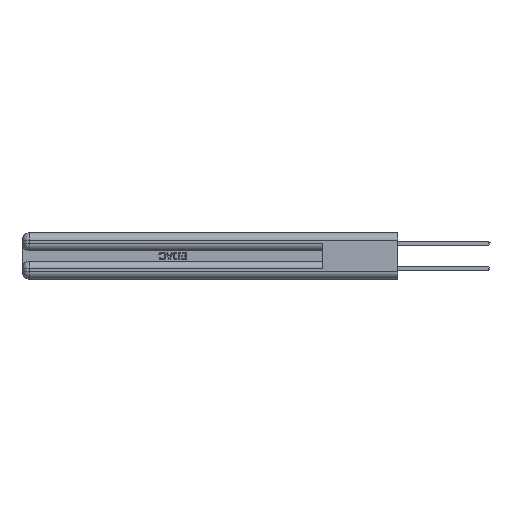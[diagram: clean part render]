
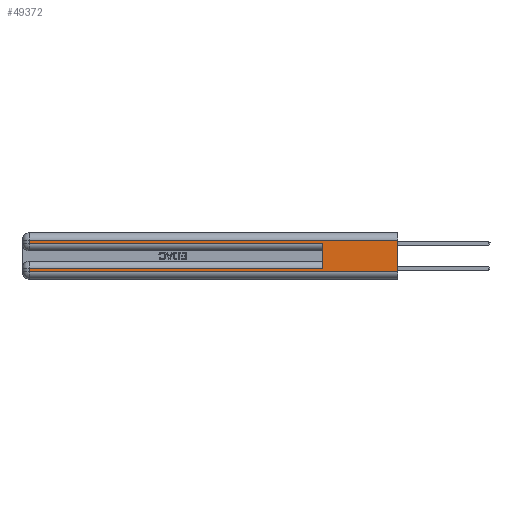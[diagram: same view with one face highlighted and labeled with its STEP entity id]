
A CAD part, left-side view. The second image highlights one B-rep face of the part: STEP entity #49372.
In plain terms, the highlighted planar face has unit normal (-1, 0, 0).
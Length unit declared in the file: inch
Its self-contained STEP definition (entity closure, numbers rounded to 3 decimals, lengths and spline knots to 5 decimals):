
#374 = EDGE_CURVE ( 'NONE', #12923, #14747, #52393, .T. ) ;
#534 = EDGE_CURVE ( 'NONE', #12923, #925, #26849, .T. ) ;
#585 = CARTESIAN_POINT ( 'NONE',  ( 0., 0., 0.37 ) ) ;
#694 = VECTOR ( 'NONE', #835, 39.37008 ) ;
#835 = DIRECTION ( 'NONE',  ( 0., 0., -1. ) ) ;
#925 = VERTEX_POINT ( 'NONE', #38892 ) ;
#1058 = LINE ( 'NONE', #45778, #47148 ) ;
#1672 = DIRECTION ( 'NONE',  ( 0., -1., 0. ) ) ;
#3564 = DIRECTION ( 'NONE',  ( 0., 1., 0. ) ) ;
#4572 = CARTESIAN_POINT ( 'NONE',  ( 0., 2.94, 0.37 ) ) ;
#5082 = CARTESIAN_POINT ( 'NONE',  ( 0., 0., 0.31 ) ) ;
#5516 = EDGE_CURVE ( 'NONE', #925, #50836, #44206, .T. ) ;
#7382 = DIRECTION ( 'NONE',  ( 0., 1., 0. ) ) ;
#8283 = VECTOR ( 'NONE', #7382, 39.37008 ) ;
#8948 = VECTOR ( 'NONE', #32881, 39.37008 ) ;
#10484 = ORIENTED_EDGE ( 'NONE', *, *, #16771, .F. ) ;
#10670 = EDGE_CURVE ( 'NONE', #12885, #26921, #10829, .T. ) ;
#10829 = LINE ( 'NONE', #48444, #51081 ) ;
#10860 = VECTOR ( 'NONE', #1672, 39.37008 ) ;
#12379 = EDGE_CURVE ( 'NONE', #45202, #14747, #41952, .T. ) ;
#12885 = VERTEX_POINT ( 'NONE', #21507 ) ;
#12923 = VERTEX_POINT ( 'NONE', #17211 ) ;
#13219 = ORIENTED_EDGE ( 'NONE', *, *, #44839, .T. ) ;
#14747 = VERTEX_POINT ( 'NONE', #28110 ) ;
#16771 = EDGE_CURVE ( 'NONE', #12885, #24534, #1058, .T. ) ;
#17211 = CARTESIAN_POINT ( 'NONE',  ( 0., 0., 0.31 ) ) ;
#17705 = ORIENTED_EDGE ( 'NONE', *, *, #12379, .T. ) ;
#18285 = ORIENTED_EDGE ( 'NONE', *, *, #374, .F. ) ;
#18946 = VECTOR ( 'NONE', #51471, 39.37008 ) ;
#20356 = FACE_OUTER_BOUND ( 'NONE', #47467, .T. ) ;
#21507 = CARTESIAN_POINT ( 'NONE',  ( 0., 0.6, 0.085 ) ) ;
#22694 = CARTESIAN_POINT ( 'NONE',  ( 0., 0.6, 0.285 ) ) ;
#24534 = VERTEX_POINT ( 'NONE', #22694 ) ;
#26626 = AXIS2_PLACEMENT_3D ( 'NONE', #44166, #43993, #52196 ) ;
#26849 = LINE ( 'NONE', #5082, #8283 ) ;
#26921 = VERTEX_POINT ( 'NONE', #37259 ) ;
#28110 = CARTESIAN_POINT ( 'NONE',  ( 0., 0., 0.06 ) ) ;
#29400 = LINE ( 'NONE', #29724, #36427 ) ;
#29718 = CARTESIAN_POINT ( 'NONE',  ( 0., 0., 0.285 ) ) ;
#29724 = CARTESIAN_POINT ( 'NONE',  ( 0., 2.94, 0.37 ) ) ;
#30258 = ORIENTED_EDGE ( 'NONE', *, *, #534, .T. ) ;
#30771 = ORIENTED_EDGE ( 'NONE', *, *, #48522, .T. ) ;
#32127 = ORIENTED_EDGE ( 'NONE', *, *, #5516, .T. ) ;
#32140 = PLANE ( 'NONE',  #26626 ) ;
#32881 = DIRECTION ( 'NONE',  ( 0., 0., -1. ) ) ;
#33396 = DIRECTION ( 'NONE',  ( 0., 0., 1. ) ) ;
#34644 = CARTESIAN_POINT ( 'NONE',  ( 0., 2.94, 0.285 ) ) ;
#36427 = VECTOR ( 'NONE', #38298, 39.37008 ) ;
#37259 = CARTESIAN_POINT ( 'NONE',  ( 0., 2.94, 0.085 ) ) ;
#38298 = DIRECTION ( 'NONE',  ( 0., 0., -1. ) ) ;
#38892 = CARTESIAN_POINT ( 'NONE',  ( 0., 2.94, 0.31 ) ) ;
#40889 = LINE ( 'NONE', #29718, #10860 ) ;
#41952 = LINE ( 'NONE', #51295, #18946 ) ;
#43993 = DIRECTION ( 'NONE',  ( 1., 0., 0. ) ) ;
#44166 = CARTESIAN_POINT ( 'NONE',  ( 0., 0., 0.37 ) ) ;
#44206 = LINE ( 'NONE', #4572, #694 ) ;
#44839 = EDGE_CURVE ( 'NONE', #26921, #45202, #29400, .T. ) ;
#45202 = VERTEX_POINT ( 'NONE', #48159 ) ;
#45778 = CARTESIAN_POINT ( 'NONE',  ( 0., 0.6, 0.145 ) ) ;
#47148 = VECTOR ( 'NONE', #33396, 39.37008 ) ;
#47467 = EDGE_LOOP ( 'NONE', ( #18285, #30258, #32127, #30771, #10484, #47619, #13219, #17705 ) ) ;
#47619 = ORIENTED_EDGE ( 'NONE', *, *, #10670, .T. ) ;
#48159 = CARTESIAN_POINT ( 'NONE',  ( 0., 2.94, 0.06 ) ) ;
#48444 = CARTESIAN_POINT ( 'NONE',  ( 0., 0., 0.085 ) ) ;
#48522 = EDGE_CURVE ( 'NONE', #50836, #24534, #40889, .T. ) ;
#49372 = ADVANCED_FACE ( 'NONE', ( #20356 ), #32140, .F. ) ;
#50836 = VERTEX_POINT ( 'NONE', #34644 ) ;
#51081 = VECTOR ( 'NONE', #3564, 39.37008 ) ;
#51295 = CARTESIAN_POINT ( 'NONE',  ( 0., 0., 0.06 ) ) ;
#51471 = DIRECTION ( 'NONE',  ( 0., -1., 0. ) ) ;
#52196 = DIRECTION ( 'NONE',  ( 0., 0., -1. ) ) ;
#52393 = LINE ( 'NONE', #585, #8948 ) ;
